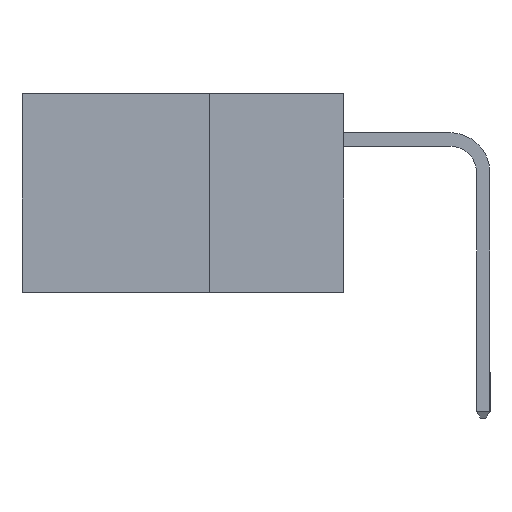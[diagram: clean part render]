
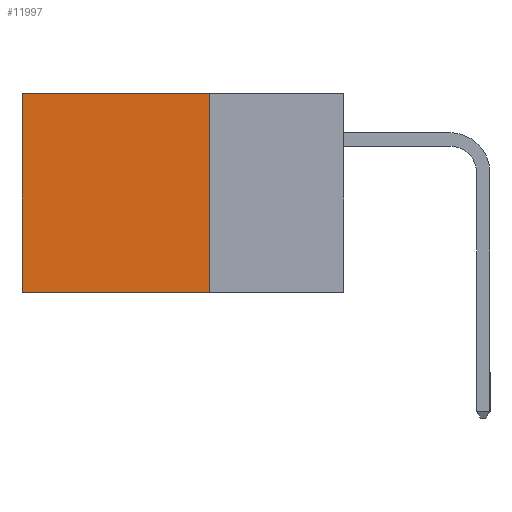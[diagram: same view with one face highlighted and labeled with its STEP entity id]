
A CAD part, left-side view. The second image highlights one B-rep face of the part: STEP entity #11997.
In plain terms, the highlighted planar face has unit normal (-1, 0, 0).
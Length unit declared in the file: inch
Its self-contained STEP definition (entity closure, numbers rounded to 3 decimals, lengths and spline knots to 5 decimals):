
#503 = VERTEX_POINT ( 'NONE', #7582 ) ;
#1781 = VERTEX_POINT ( 'NONE', #7452 ) ;
#2079 = DIRECTION ( 'NONE',  ( 1., 0., 0. ) ) ;
#2183 = DIRECTION ( 'NONE',  ( 0., 0., -1. ) ) ;
#2472 = CARTESIAN_POINT ( 'NONE',  ( 0.2615, 0.6, -0.37 ) ) ;
#2752 = EDGE_CURVE ( 'NONE', #503, #12848, #4821, .T. ) ;
#3061 = ORIENTED_EDGE ( 'NONE', *, *, #5187, .F. ) ;
#3087 = FACE_OUTER_BOUND ( 'NONE', #7135, .T. ) ;
#3920 = PLANE ( 'NONE',  #12641 ) ;
#3940 = DIRECTION ( 'NONE',  ( 0., 1., 0. ) ) ;
#4002 = LINE ( 'NONE', #13235, #6909 ) ;
#4094 = CARTESIAN_POINT ( 'NONE',  ( 0.2615, 0.25, -0.37 ) ) ;
#4178 = ORIENTED_EDGE ( 'NONE', *, *, #2752, .F. ) ;
#4821 = LINE ( 'NONE', #8862, #8189 ) ;
#5187 = EDGE_CURVE ( 'NONE', #12848, #6936, #4002, .T. ) ;
#5574 = LINE ( 'NONE', #5643, #11978 ) ;
#5643 = CARTESIAN_POINT ( 'NONE',  ( 0.2615, 0.25, 0. ) ) ;
#6685 = DIRECTION ( 'NONE',  ( 0., 1., 0. ) ) ;
#6909 = VECTOR ( 'NONE', #3940, 39.37008 ) ;
#6936 = VERTEX_POINT ( 'NONE', #2472 ) ;
#7135 = EDGE_LOOP ( 'NONE', ( #9843, #3061, #4178, #8616 ) ) ;
#7173 = CARTESIAN_POINT ( 'NONE',  ( 0.2615, 0.25, -0.37 ) ) ;
#7452 = CARTESIAN_POINT ( 'NONE',  ( 0.2615, 0.6, 0. ) ) ;
#7582 = CARTESIAN_POINT ( 'NONE',  ( 0.2615, 0.25, 0. ) ) ;
#8189 = VECTOR ( 'NONE', #9676, 39.37008 ) ;
#8284 = VECTOR ( 'NONE', #2183, 39.37008 ) ;
#8407 = EDGE_CURVE ( 'NONE', #1781, #6936, #9241, .T. ) ;
#8616 = ORIENTED_EDGE ( 'NONE', *, *, #9974, .T. ) ;
#8862 = CARTESIAN_POINT ( 'NONE',  ( 0.2615, 0.25, -0.37 ) ) ;
#8984 = DIRECTION ( 'NONE',  ( 0., 0., -1. ) ) ;
#9241 = LINE ( 'NONE', #10444, #8284 ) ;
#9676 = DIRECTION ( 'NONE',  ( 0., 0., -1. ) ) ;
#9843 = ORIENTED_EDGE ( 'NONE', *, *, #8407, .T. ) ;
#9974 = EDGE_CURVE ( 'NONE', #503, #1781, #5574, .T. ) ;
#10444 = CARTESIAN_POINT ( 'NONE',  ( 0.2615, 0.6, -0.37 ) ) ;
#11978 = VECTOR ( 'NONE', #6685, 39.37008 ) ;
#11997 = ADVANCED_FACE ( 'NONE', ( #3087 ), #3920, .F. ) ;
#12641 = AXIS2_PLACEMENT_3D ( 'NONE', #7173, #2079, #8984 ) ;
#12848 = VERTEX_POINT ( 'NONE', #4094 ) ;
#13235 = CARTESIAN_POINT ( 'NONE',  ( 0.2615, 0.25, -0.37 ) ) ;
